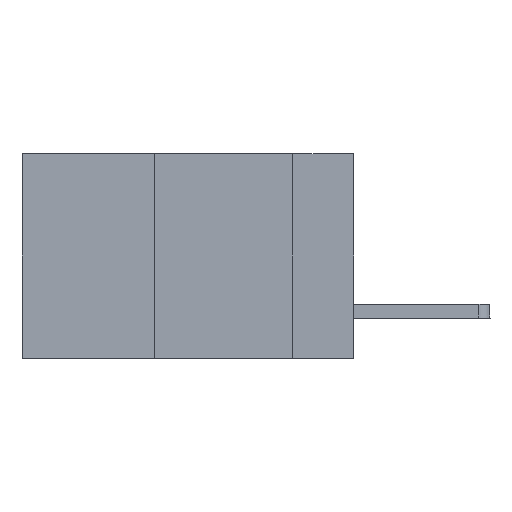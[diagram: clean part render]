
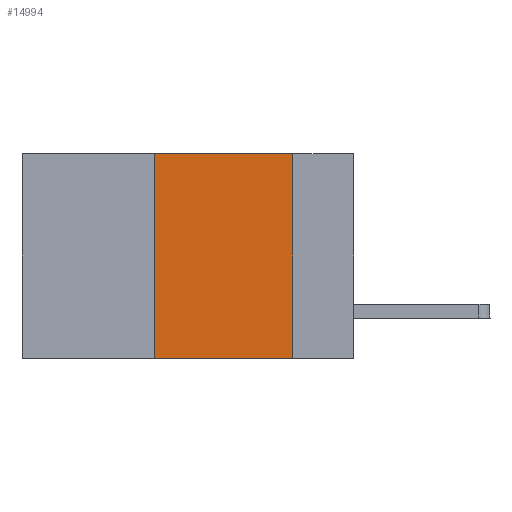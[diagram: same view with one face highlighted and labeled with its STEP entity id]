
A CAD part, left-side view. The second image highlights one B-rep face of the part: STEP entity #14994.
In plain terms, the highlighted planar face has unit normal (-1, 0, 0).
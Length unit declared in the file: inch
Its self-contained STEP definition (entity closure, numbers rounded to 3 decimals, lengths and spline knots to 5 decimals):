
#47 = EDGE_LOOP ( 'NONE', ( #430, #11247, #10137, #13250 ) ) ;
#430 = ORIENTED_EDGE ( 'NONE', *, *, #3199, .F. ) ;
#507 = PLANE ( 'NONE',  #2947 ) ;
#1128 = LINE ( 'NONE', #7637, #10437 ) ;
#1999 = LINE ( 'NONE', #5861, #2408 ) ;
#2408 = VECTOR ( 'NONE', #10603, 39.37008 ) ;
#2947 = AXIS2_PLACEMENT_3D ( 'NONE', #14908, #9004, #9054 ) ;
#3199 = EDGE_CURVE ( 'NONE', #15487, #6257, #1128, .T. ) ;
#3255 = CARTESIAN_POINT ( 'NONE',  ( 0., 0.11, -0.37 ) ) ;
#3268 = CARTESIAN_POINT ( 'NONE',  ( 0., 0.36, 0. ) ) ;
#4697 = EDGE_CURVE ( 'NONE', #11050, #6257, #14284, .T. ) ;
#5108 = EDGE_CURVE ( 'NONE', #11050, #14510, #14267, .T. ) ;
#5684 = FACE_OUTER_BOUND ( 'NONE', #47, .T. ) ;
#5861 = CARTESIAN_POINT ( 'NONE',  ( 0., 0.6, 0. ) ) ;
#5929 = VECTOR ( 'NONE', #6040, 39.37008 ) ;
#6040 = DIRECTION ( 'NONE',  ( 0., 0., 1. ) ) ;
#6211 = DIRECTION ( 'NONE',  ( 0., -1., 0. ) ) ;
#6257 = VERTEX_POINT ( 'NONE', #3255 ) ;
#7589 = CARTESIAN_POINT ( 'NONE',  ( 0., 0.11, 0. ) ) ;
#7637 = CARTESIAN_POINT ( 'NONE',  ( 0., 0.11, 0. ) ) ;
#8819 = DIRECTION ( 'NONE',  ( 0., 0., -1. ) ) ;
#9004 = DIRECTION ( 'NONE',  ( 1., 0., 0. ) ) ;
#9054 = DIRECTION ( 'NONE',  ( 0., 0., -1. ) ) ;
#9862 = CARTESIAN_POINT ( 'NONE',  ( 0., 0.6, -0.37 ) ) ;
#10137 = ORIENTED_EDGE ( 'NONE', *, *, #5108, .F. ) ;
#10437 = VECTOR ( 'NONE', #8819, 39.37008 ) ;
#10603 = DIRECTION ( 'NONE',  ( 0., -1., 0. ) ) ;
#10783 = VECTOR ( 'NONE', #6211, 39.37008 ) ;
#11050 = VERTEX_POINT ( 'NONE', #12852 ) ;
#11247 = ORIENTED_EDGE ( 'NONE', *, *, #14609, .F. ) ;
#12852 = CARTESIAN_POINT ( 'NONE',  ( 0., 0.36, -0.37 ) ) ;
#13250 = ORIENTED_EDGE ( 'NONE', *, *, #4697, .T. ) ;
#14267 = LINE ( 'NONE', #14330, #5929 ) ;
#14284 = LINE ( 'NONE', #9862, #10783 ) ;
#14330 = CARTESIAN_POINT ( 'NONE',  ( 0., 0.36, 0. ) ) ;
#14510 = VERTEX_POINT ( 'NONE', #3268 ) ;
#14609 = EDGE_CURVE ( 'NONE', #14510, #15487, #1999, .T. ) ;
#14908 = CARTESIAN_POINT ( 'NONE',  ( 0., 0.6, 0. ) ) ;
#14994 = ADVANCED_FACE ( 'NONE', ( #5684 ), #507, .F. ) ;
#15487 = VERTEX_POINT ( 'NONE', #7589 ) ;
